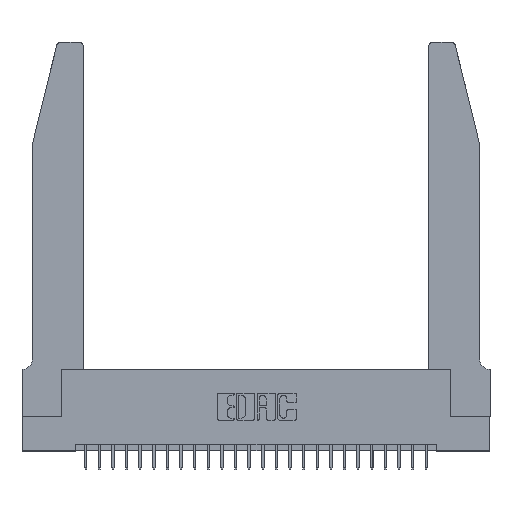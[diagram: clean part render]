
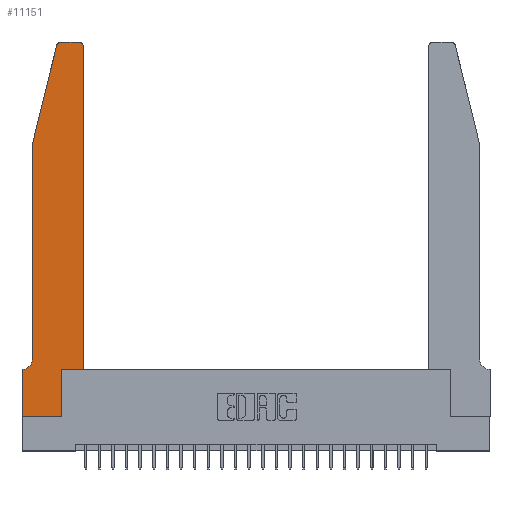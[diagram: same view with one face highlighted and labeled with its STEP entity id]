
A CAD part, top view. The second image highlights one B-rep face of the part: STEP entity #11151.
In plain terms, the highlighted planar face has unit normal (0, 0, 1).
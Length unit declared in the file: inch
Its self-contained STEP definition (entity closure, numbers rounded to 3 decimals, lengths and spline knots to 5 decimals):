
#140 = DIRECTION ( 'NONE',  ( 0., 0., -1. ) ) ;
#371 = VERTEX_POINT ( 'NONE', #21121 ) ;
#493 = DIRECTION ( 'NONE',  ( 1., 0., 0. ) ) ;
#888 = DIRECTION ( 'NONE',  ( -1., 0., 0. ) ) ;
#998 = DIRECTION ( 'NONE',  ( -1., 0., 0. ) ) ;
#1656 = CARTESIAN_POINT ( 'NONE',  ( 0.4205, 2.72, 0.37 ) ) ;
#1877 = CARTESIAN_POINT ( 'NONE',  ( 0., 0., 0.37 ) ) ;
#2479 = CIRCLE ( 'NONE', #10044, 0.07 ) ;
#3077 = VERTEX_POINT ( 'NONE', #4189 ) ;
#3307 = CARTESIAN_POINT ( 'NONE',  ( 0.4205, 2.75, 0.37 ) ) ;
#3325 = VECTOR ( 'NONE', #17593, 39.37008 ) ;
#3372 = VERTEX_POINT ( 'NONE', #3307 ) ;
#3439 = ORIENTED_EDGE ( 'NONE', *, *, #26914, .T. ) ;
#3786 = EDGE_CURVE ( 'NONE', #3077, #17144, #11611, .T. ) ;
#3842 = LINE ( 'NONE', #1877, #15646 ) ;
#4189 = CARTESIAN_POINT ( 'NONE',  ( 0.0055, 0.35, 0.37 ) ) ;
#4298 = EDGE_CURVE ( 'NONE', #371, #5097, #11232, .T. ) ;
#4338 = CARTESIAN_POINT ( 'NONE',  ( 0.2865, 0.35, 0.37 ) ) ;
#4677 = LINE ( 'NONE', #10664, #5551 ) ;
#5042 = CARTESIAN_POINT ( 'NONE',  ( 0.2605, 2.75, 0.37 ) ) ;
#5097 = VERTEX_POINT ( 'NONE', #23402 ) ;
#5551 = VECTOR ( 'NONE', #493, 39.37008 ) ;
#5600 = ORIENTED_EDGE ( 'NONE', *, *, #18782, .T. ) ;
#5977 = VECTOR ( 'NONE', #888, 39.37008 ) ;
#5999 = VERTEX_POINT ( 'NONE', #25642 ) ;
#6090 = VERTEX_POINT ( 'NONE', #6623 ) ;
#6113 = LINE ( 'NONE', #16376, #19734 ) ;
#6620 = VECTOR ( 'NONE', #9736, 39.37008 ) ;
#6623 = CARTESIAN_POINT ( 'NONE',  ( 0.2865, 0., 0.37 ) ) ;
#7551 = ORIENTED_EDGE ( 'NONE', *, *, #25331, .T. ) ;
#7629 = ORIENTED_EDGE ( 'NONE', *, *, #25008, .T. ) ;
#8187 = PLANE ( 'NONE',  #22121 ) ;
#9076 = AXIS2_PLACEMENT_3D ( 'NONE', #27374, #21119, #10451 ) ;
#9384 = CARTESIAN_POINT ( 'NONE',  ( 0.0755, 0.35, 0.37 ) ) ;
#9736 = DIRECTION ( 'NONE',  ( 0., 1., 0. ) ) ;
#9834 = VERTEX_POINT ( 'NONE', #25763 ) ;
#9848 = CARTESIAN_POINT ( 'NONE',  ( 0.4505, 0.35, 0.37 ) ) ;
#10044 = AXIS2_PLACEMENT_3D ( 'NONE', #15083, #140, #14951 ) ;
#10421 = CARTESIAN_POINT ( 'NONE',  ( 0., 0.35, 0.37 ) ) ;
#10451 = DIRECTION ( 'NONE',  ( 1., 0., 0. ) ) ;
#10632 = DIRECTION ( 'NONE',  ( 0., -1., 0. ) ) ;
#10664 = CARTESIAN_POINT ( 'NONE',  ( 0.4505, 0.35, 0.37 ) ) ;
#10732 = CARTESIAN_POINT ( 'NONE',  ( 0.4505, 2.72, 0.37 ) ) ;
#10962 = CARTESIAN_POINT ( 'NONE',  ( 0.4505, 0.35, 0.37 ) ) ;
#11151 = ADVANCED_FACE ( 'NONE', ( #18741 ), #8187, .T. ) ;
#11232 = LINE ( 'NONE', #13424, #3325 ) ;
#11234 = DIRECTION ( 'NONE',  ( 0., 1., 0. ) ) ;
#11611 = LINE ( 'NONE', #9384, #5977 ) ;
#12084 = VERTEX_POINT ( 'NONE', #26179 ) ;
#12092 = DIRECTION ( 'NONE',  ( 0., -1., 0. ) ) ;
#12151 = CIRCLE ( 'NONE', #9076, 0.03 ) ;
#12618 = ORIENTED_EDGE ( 'NONE', *, *, #17786, .T. ) ;
#13120 = CARTESIAN_POINT ( 'NONE',  ( 0., 0.35, 0.37 ) ) ;
#13165 = LINE ( 'NONE', #10962, #20201 ) ;
#13424 = CARTESIAN_POINT ( 'NONE',  ( 0.0755, 2., 0.37 ) ) ;
#13925 = ORIENTED_EDGE ( 'NONE', *, *, #27057, .T. ) ;
#14116 = ORIENTED_EDGE ( 'NONE', *, *, #4298, .T. ) ;
#14951 = DIRECTION ( 'NONE',  ( -1., 0., 0. ) ) ;
#15083 = CARTESIAN_POINT ( 'NONE',  ( 0.0055, 0.42, 0.37 ) ) ;
#15289 = CARTESIAN_POINT ( 'NONE',  ( 0., 0., 0.37 ) ) ;
#15613 = ORIENTED_EDGE ( 'NONE', *, *, #26223, .T. ) ;
#15646 = VECTOR ( 'NONE', #10632, 39.37008 ) ;
#15945 = VECTOR ( 'NONE', #23666, 39.37008 ) ;
#16376 = CARTESIAN_POINT ( 'NONE',  ( 0.0755, 2., 0.37 ) ) ;
#16603 = EDGE_CURVE ( 'NONE', #26632, #3372, #26988, .T. ) ;
#16645 = DIRECTION ( 'NONE',  ( 0., 0., 1. ) ) ;
#17104 = VERTEX_POINT ( 'NONE', #9848 ) ;
#17144 = VERTEX_POINT ( 'NONE', #13120 ) ;
#17593 = DIRECTION ( 'NONE',  ( -0.239, -0.971, 0. ) ) ;
#17640 = AXIS2_PLACEMENT_3D ( 'NONE', #1656, #26942, #22632 ) ;
#17786 = EDGE_CURVE ( 'NONE', #6090, #20730, #26526, .T. ) ;
#18741 = FACE_OUTER_BOUND ( 'NONE', #19568, .T. ) ;
#18782 = EDGE_CURVE ( 'NONE', #5999, #6090, #19477, .T. ) ;
#18870 = DIRECTION ( 'NONE',  ( 1., 0., 0. ) ) ;
#18895 = ORIENTED_EDGE ( 'NONE', *, *, #27029, .T. ) ;
#19376 = ORIENTED_EDGE ( 'NONE', *, *, #16603, .T. ) ;
#19477 = LINE ( 'NONE', #15289, #15945 ) ;
#19568 = EDGE_LOOP ( 'NONE', ( #20426, #7551, #14116, #3439, #13925, #22440, #7629, #5600, #12618, #15613, #18895, #19376 ) ) ;
#19734 = VECTOR ( 'NONE', #12092, 39.37008 ) ;
#20201 = VECTOR ( 'NONE', #11234, 39.37008 ) ;
#20426 = ORIENTED_EDGE ( 'NONE', *, *, #25207, .T. ) ;
#20730 = VERTEX_POINT ( 'NONE', #4338 ) ;
#21119 = DIRECTION ( 'NONE',  ( 0., 0., 1. ) ) ;
#21121 = CARTESIAN_POINT ( 'NONE',  ( 0.25487, 2.72718, 0.37 ) ) ;
#22121 = AXIS2_PLACEMENT_3D ( 'NONE', #10421, #16645, #18870 ) ;
#22440 = ORIENTED_EDGE ( 'NONE', *, *, #3786, .T. ) ;
#22632 = DIRECTION ( 'NONE',  ( 1., 0., 0. ) ) ;
#23402 = CARTESIAN_POINT ( 'NONE',  ( 0.0755, 2., 0.37 ) ) ;
#23666 = DIRECTION ( 'NONE',  ( 1., 0., 0. ) ) ;
#24139 = VECTOR ( 'NONE', #998, 39.37008 ) ;
#24450 = CARTESIAN_POINT ( 'NONE',  ( 0.2865, 0.35, 0.37 ) ) ;
#25008 = EDGE_CURVE ( 'NONE', #17144, #5999, #3842, .T. ) ;
#25207 = EDGE_CURVE ( 'NONE', #3372, #12084, #26706, .T. ) ;
#25331 = EDGE_CURVE ( 'NONE', #12084, #371, #12151, .T. ) ;
#25642 = CARTESIAN_POINT ( 'NONE',  ( 0., 0., 0.37 ) ) ;
#25763 = CARTESIAN_POINT ( 'NONE',  ( 0.0755, 0.42, 0.37 ) ) ;
#26179 = CARTESIAN_POINT ( 'NONE',  ( 0.284, 2.75, 0.37 ) ) ;
#26223 = EDGE_CURVE ( 'NONE', #20730, #17104, #4677, .T. ) ;
#26526 = LINE ( 'NONE', #24450, #6620 ) ;
#26632 = VERTEX_POINT ( 'NONE', #10732 ) ;
#26706 = LINE ( 'NONE', #5042, #24139 ) ;
#26914 = EDGE_CURVE ( 'NONE', #5097, #9834, #6113, .T. ) ;
#26942 = DIRECTION ( 'NONE',  ( 0., 0., 1. ) ) ;
#26988 = CIRCLE ( 'NONE', #17640, 0.03 ) ;
#27029 = EDGE_CURVE ( 'NONE', #17104, #26632, #13165, .T. ) ;
#27057 = EDGE_CURVE ( 'NONE', #9834, #3077, #2479, .T. ) ;
#27374 = CARTESIAN_POINT ( 'NONE',  ( 0.284, 2.72, 0.37 ) ) ;
